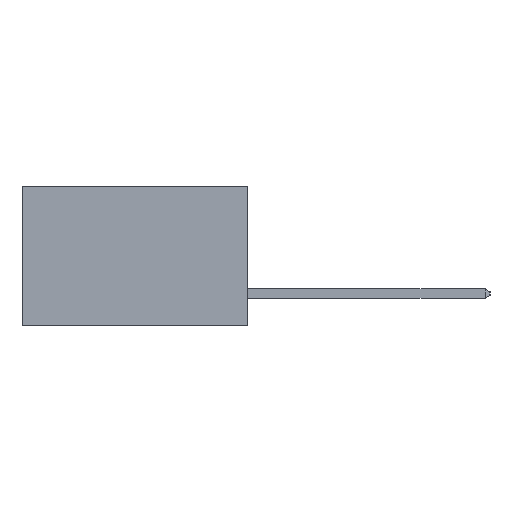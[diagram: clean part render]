
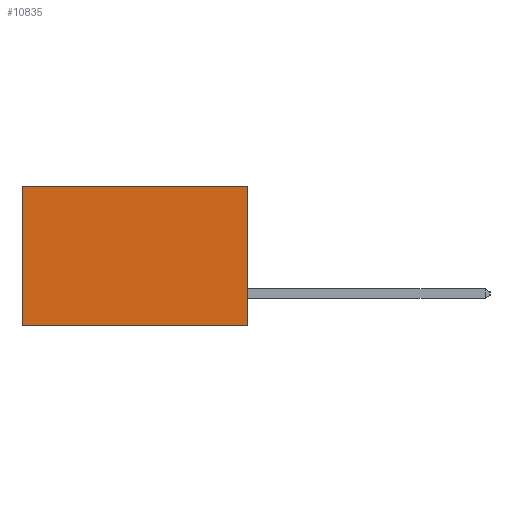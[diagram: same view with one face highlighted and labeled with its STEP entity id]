
A CAD part, left-side view. The second image highlights one B-rep face of the part: STEP entity #10835.
In plain terms, the highlighted planar face has unit normal (-1, 0, 0).
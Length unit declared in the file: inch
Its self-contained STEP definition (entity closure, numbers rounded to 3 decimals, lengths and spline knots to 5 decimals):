
#372 = CARTESIAN_POINT ( 'NONE',  ( 0.2615, 0., 0. ) ) ;
#764 = DIRECTION ( 'NONE',  ( 1., 0., 0. ) ) ;
#1011 = FACE_OUTER_BOUND ( 'NONE', #8597, .T. ) ;
#1063 = VERTEX_POINT ( 'NONE', #5540 ) ;
#1169 = LINE ( 'NONE', #12066, #9491 ) ;
#1370 = VECTOR ( 'NONE', #12628, 39.37008 ) ;
#2289 = CARTESIAN_POINT ( 'NONE',  ( 0.2615, 0., 0. ) ) ;
#2557 = CARTESIAN_POINT ( 'NONE',  ( 0.2615, 0., -0.37 ) ) ;
#3010 = VECTOR ( 'NONE', #12681, 39.37008 ) ;
#3038 = VERTEX_POINT ( 'NONE', #7879 ) ;
#4370 = ORIENTED_EDGE ( 'NONE', *, *, #4704, .F. ) ;
#4704 = EDGE_CURVE ( 'NONE', #9820, #1063, #9382, .T. ) ;
#4713 = ORIENTED_EDGE ( 'NONE', *, *, #9285, .T. ) ;
#5310 = VERTEX_POINT ( 'NONE', #10247 ) ;
#5540 = CARTESIAN_POINT ( 'NONE',  ( 0.2615, 0., -0.37 ) ) ;
#5884 = CARTESIAN_POINT ( 'NONE',  ( 0.2615, 0., -0.37 ) ) ;
#6226 = DIRECTION ( 'NONE',  ( 0., 0., -1. ) ) ;
#6308 = LINE ( 'NONE', #11752, #3010 ) ;
#6516 = DIRECTION ( 'NONE',  ( 0., 1., 0. ) ) ;
#7832 = DIRECTION ( 'NONE',  ( 0., 0., -1. ) ) ;
#7879 = CARTESIAN_POINT ( 'NONE',  ( 0.2615, 0.6, -0.37 ) ) ;
#7991 = ORIENTED_EDGE ( 'NONE', *, *, #10252, .F. ) ;
#8285 = ORIENTED_EDGE ( 'NONE', *, *, #11031, .T. ) ;
#8597 = EDGE_LOOP ( 'NONE', ( #8285, #7991, #4370, #4713 ) ) ;
#9285 = EDGE_CURVE ( 'NONE', #9820, #5310, #12290, .T. ) ;
#9382 = LINE ( 'NONE', #2557, #1370 ) ;
#9417 = VECTOR ( 'NONE', #6516, 39.37008 ) ;
#9491 = VECTOR ( 'NONE', #6226, 39.37008 ) ;
#9820 = VERTEX_POINT ( 'NONE', #2289 ) ;
#10247 = CARTESIAN_POINT ( 'NONE',  ( 0.2615, 0.6, 0. ) ) ;
#10252 = EDGE_CURVE ( 'NONE', #1063, #3038, #6308, .T. ) ;
#10835 = ADVANCED_FACE ( 'NONE', ( #1011 ), #12665, .F. ) ;
#11031 = EDGE_CURVE ( 'NONE', #5310, #3038, #1169, .T. ) ;
#11752 = CARTESIAN_POINT ( 'NONE',  ( 0.2615, 0., -0.37 ) ) ;
#12066 = CARTESIAN_POINT ( 'NONE',  ( 0.2615, 0.6, -0.37 ) ) ;
#12290 = LINE ( 'NONE', #372, #9417 ) ;
#12419 = AXIS2_PLACEMENT_3D ( 'NONE', #5884, #764, #7832 ) ;
#12628 = DIRECTION ( 'NONE',  ( 0., 0., -1. ) ) ;
#12665 = PLANE ( 'NONE',  #12419 ) ;
#12681 = DIRECTION ( 'NONE',  ( 0., 1., 0. ) ) ;
